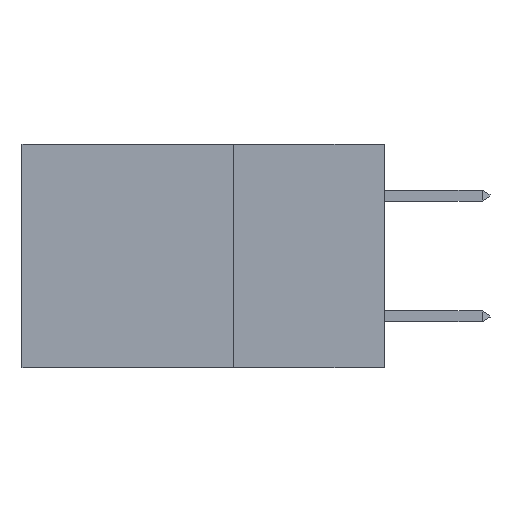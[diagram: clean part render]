
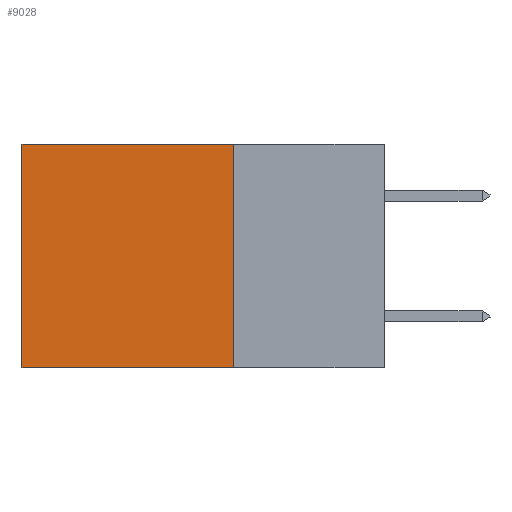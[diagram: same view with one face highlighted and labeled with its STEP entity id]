
A CAD part, left-side view. The second image highlights one B-rep face of the part: STEP entity #9028.
In plain terms, the highlighted planar face has unit normal (-1, 0, 0).
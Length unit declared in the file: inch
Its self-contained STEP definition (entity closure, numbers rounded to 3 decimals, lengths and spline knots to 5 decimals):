
#126 = CARTESIAN_POINT ( 'NONE',  ( 0.2875, 0.6, 0. ) ) ;
#190 = EDGE_CURVE ( 'NONE', #759, #6931, #5874, .T. ) ;
#264 = VERTEX_POINT ( 'NONE', #6362 ) ;
#546 = EDGE_CURVE ( 'NONE', #264, #10537, #9875, .T. ) ;
#664 = LINE ( 'NONE', #10365, #2883 ) ;
#759 = VERTEX_POINT ( 'NONE', #3309 ) ;
#1215 = EDGE_CURVE ( 'NONE', #264, #759, #664, .T. ) ;
#1751 = EDGE_LOOP ( 'NONE', ( #6304, #10407, #3658, #8036 ) ) ;
#2178 = CARTESIAN_POINT ( 'NONE',  ( 0.2875, 0.25, 0. ) ) ;
#2226 = PLANE ( 'NONE',  #3795 ) ;
#2623 = EDGE_CURVE ( 'NONE', #10537, #6931, #9965, .T. ) ;
#2883 = VECTOR ( 'NONE', #9416, 39.37008 ) ;
#3156 = DIRECTION ( 'NONE',  ( 1., 0., 0. ) ) ;
#3309 = CARTESIAN_POINT ( 'NONE',  ( 0.2875, 0.25, -0.37 ) ) ;
#3479 = VECTOR ( 'NONE', #7892, 39.37008 ) ;
#3658 = ORIENTED_EDGE ( 'NONE', *, *, #1215, .F. ) ;
#3795 = AXIS2_PLACEMENT_3D ( 'NONE', #2178, #3156, #9398 ) ;
#4592 = CARTESIAN_POINT ( 'NONE',  ( 0.2875, 0.6, -0.37 ) ) ;
#4614 = DIRECTION ( 'NONE',  ( 0., 1., 0. ) ) ;
#4825 = CARTESIAN_POINT ( 'NONE',  ( 0.2875, 0.25, 0. ) ) ;
#4845 = VECTOR ( 'NONE', #4614, 39.37008 ) ;
#4934 = VECTOR ( 'NONE', #11043, 39.37008 ) ;
#5874 = LINE ( 'NONE', #7194, #3479 ) ;
#6304 = ORIENTED_EDGE ( 'NONE', *, *, #2623, .T. ) ;
#6362 = CARTESIAN_POINT ( 'NONE',  ( 0.2875, 0.25, 0. ) ) ;
#6931 = VERTEX_POINT ( 'NONE', #4592 ) ;
#7194 = CARTESIAN_POINT ( 'NONE',  ( 0.2875, 0.25, -0.37 ) ) ;
#7892 = DIRECTION ( 'NONE',  ( 0., 1., 0. ) ) ;
#8036 = ORIENTED_EDGE ( 'NONE', *, *, #546, .T. ) ;
#9028 = ADVANCED_FACE ( 'NONE', ( #10944 ), #2226, .F. ) ;
#9398 = DIRECTION ( 'NONE',  ( 0., 0., -1. ) ) ;
#9416 = DIRECTION ( 'NONE',  ( 0., 0., -1. ) ) ;
#9875 = LINE ( 'NONE', #4825, #4845 ) ;
#9965 = LINE ( 'NONE', #11102, #4934 ) ;
#10365 = CARTESIAN_POINT ( 'NONE',  ( 0.2875, 0.25, 0. ) ) ;
#10407 = ORIENTED_EDGE ( 'NONE', *, *, #190, .F. ) ;
#10537 = VERTEX_POINT ( 'NONE', #126 ) ;
#10944 = FACE_OUTER_BOUND ( 'NONE', #1751, .T. ) ;
#11043 = DIRECTION ( 'NONE',  ( 0., 0., -1. ) ) ;
#11102 = CARTESIAN_POINT ( 'NONE',  ( 0.2875, 0.6, 0. ) ) ;
